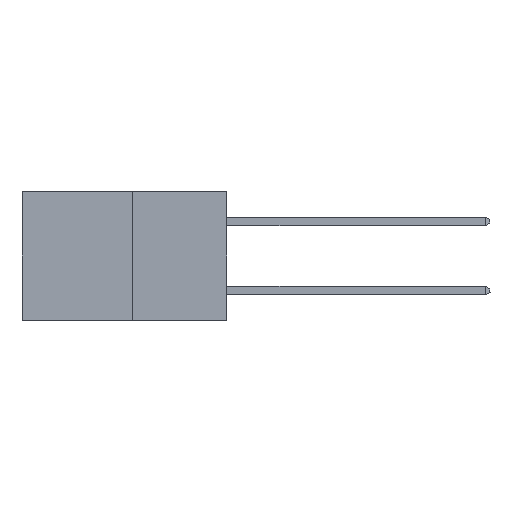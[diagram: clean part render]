
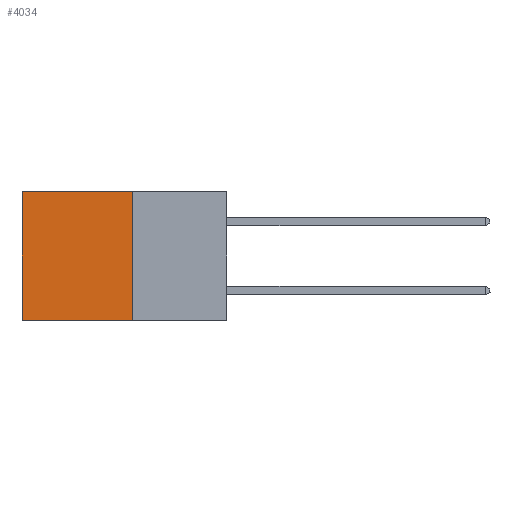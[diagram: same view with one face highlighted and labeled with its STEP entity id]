
A CAD part, left-side view. The second image highlights one B-rep face of the part: STEP entity #4034.
In plain terms, the highlighted planar face has unit normal (-1, 0, 0).
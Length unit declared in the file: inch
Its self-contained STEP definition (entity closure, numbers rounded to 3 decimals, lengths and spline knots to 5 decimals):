
#255 = LINE ( 'NONE', #12593, #9801 ) ;
#261 = VERTEX_POINT ( 'NONE', #6117 ) ;
#312 = VECTOR ( 'NONE', #7815, 39.37008 ) ;
#441 = VECTOR ( 'NONE', #13299, 39.37008 ) ;
#791 = FACE_OUTER_BOUND ( 'NONE', #9444, .T. ) ;
#984 = DIRECTION ( 'NONE',  ( 0., 1., 0. ) ) ;
#1049 = CARTESIAN_POINT ( 'NONE',  ( 0.277, 0.27, 0. ) ) ;
#1280 = ORIENTED_EDGE ( 'NONE', *, *, #9065, .F. ) ;
#1560 = VERTEX_POINT ( 'NONE', #6005 ) ;
#2934 = CARTESIAN_POINT ( 'NONE',  ( 0.277, 0.59, 0. ) ) ;
#2953 = CARTESIAN_POINT ( 'NONE',  ( 0.277, 0.27, -0.37 ) ) ;
#3151 = EDGE_CURVE ( 'NONE', #6076, #1560, #7242, .T. ) ;
#3281 = DIRECTION ( 'NONE',  ( 0., 0., -1. ) ) ;
#3468 = DIRECTION ( 'NONE',  ( 1., 0., 0. ) ) ;
#3719 = PLANE ( 'NONE',  #13184 ) ;
#3887 = CARTESIAN_POINT ( 'NONE',  ( 0.277, 0.27, -0.37 ) ) ;
#4034 = ADVANCED_FACE ( 'NONE', ( #791 ), #3719, .F. ) ;
#4793 = ORIENTED_EDGE ( 'NONE', *, *, #14651, .T. ) ;
#6005 = CARTESIAN_POINT ( 'NONE',  ( 0.277, 0.27, -0.37 ) ) ;
#6076 = VERTEX_POINT ( 'NONE', #14016 ) ;
#6117 = CARTESIAN_POINT ( 'NONE',  ( 0.277, 0.59, -0.37 ) ) ;
#6655 = EDGE_CURVE ( 'NONE', #6076, #9803, #6855, .T. ) ;
#6855 = LINE ( 'NONE', #1049, #13287 ) ;
#7242 = LINE ( 'NONE', #7760, #312 ) ;
#7760 = CARTESIAN_POINT ( 'NONE',  ( 0.277, 0.27, -0.37 ) ) ;
#7815 = DIRECTION ( 'NONE',  ( 0., 0., -1. ) ) ;
#9065 = EDGE_CURVE ( 'NONE', #1560, #261, #14178, .T. ) ;
#9444 = EDGE_LOOP ( 'NONE', ( #4793, #1280, #13352, #12498 ) ) ;
#9801 = VECTOR ( 'NONE', #13896, 39.37008 ) ;
#9803 = VERTEX_POINT ( 'NONE', #2934 ) ;
#12498 = ORIENTED_EDGE ( 'NONE', *, *, #6655, .T. ) ;
#12593 = CARTESIAN_POINT ( 'NONE',  ( 0.277, 0.59, -0.37 ) ) ;
#13184 = AXIS2_PLACEMENT_3D ( 'NONE', #3887, #3468, #3281 ) ;
#13287 = VECTOR ( 'NONE', #984, 39.37008 ) ;
#13299 = DIRECTION ( 'NONE',  ( 0., 1., 0. ) ) ;
#13352 = ORIENTED_EDGE ( 'NONE', *, *, #3151, .F. ) ;
#13896 = DIRECTION ( 'NONE',  ( 0., 0., -1. ) ) ;
#14016 = CARTESIAN_POINT ( 'NONE',  ( 0.277, 0.27, 0. ) ) ;
#14178 = LINE ( 'NONE', #2953, #441 ) ;
#14651 = EDGE_CURVE ( 'NONE', #9803, #261, #255, .T. ) ;
